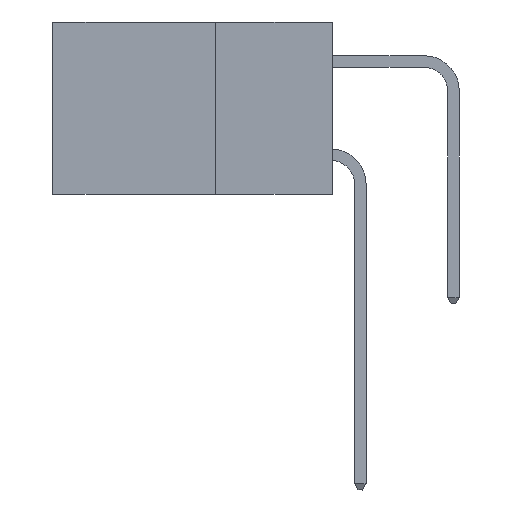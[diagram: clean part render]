
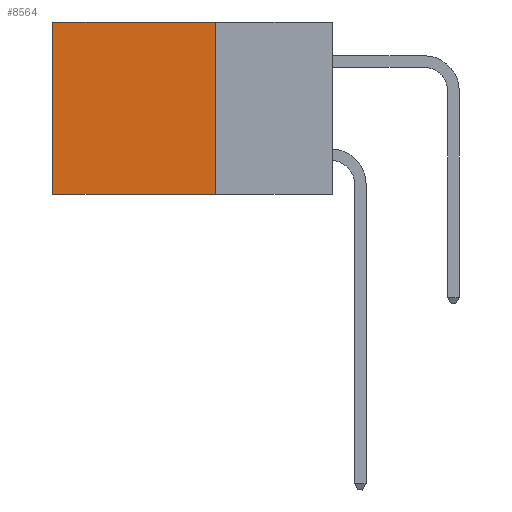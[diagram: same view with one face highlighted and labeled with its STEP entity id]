
A CAD part, left-side view. The second image highlights one B-rep face of the part: STEP entity #8564.
In plain terms, the highlighted planar face has unit normal (-1, 0, 0).
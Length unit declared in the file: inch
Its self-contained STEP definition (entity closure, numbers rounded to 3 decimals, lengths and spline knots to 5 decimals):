
#1669 = EDGE_CURVE ( 'NONE', #14055, #18018, #20801, .T. ) ;
#3012 = VERTEX_POINT ( 'NONE', #21772 ) ;
#3444 = AXIS2_PLACEMENT_3D ( 'NONE', #14337, #22350, #10398 ) ;
#4291 = PLANE ( 'NONE',  #3444 ) ;
#4457 = FACE_OUTER_BOUND ( 'NONE', #13215, .T. ) ;
#4543 = CARTESIAN_POINT ( 'NONE',  ( 0.298, 0.6, 0. ) ) ;
#6058 = CARTESIAN_POINT ( 'NONE',  ( 0.298, 0.6, -0.37 ) ) ;
#6430 = DIRECTION ( 'NONE',  ( 0., 1., 0. ) ) ;
#6864 = CARTESIAN_POINT ( 'NONE',  ( 0.298, 0.25, -0.37 ) ) ;
#7006 = LINE ( 'NONE', #14476, #21734 ) ;
#8564 = ADVANCED_FACE ( 'NONE', ( #4457 ), #4291, .F. ) ;
#8604 = EDGE_CURVE ( 'NONE', #14055, #3012, #18590, .T. ) ;
#9523 = CARTESIAN_POINT ( 'NONE',  ( 0.298, 0.25, 0. ) ) ;
#10398 = DIRECTION ( 'NONE',  ( 0., 0., -1. ) ) ;
#10543 = DIRECTION ( 'NONE',  ( 0., 1., 0. ) ) ;
#10995 = ORIENTED_EDGE ( 'NONE', *, *, #11214, .F. ) ;
#11064 = VERTEX_POINT ( 'NONE', #6058 ) ;
#11214 = EDGE_CURVE ( 'NONE', #18018, #11064, #7006, .T. ) ;
#11528 = DIRECTION ( 'NONE',  ( 0., 0., -1. ) ) ;
#11927 = ORIENTED_EDGE ( 'NONE', *, *, #1669, .F. ) ;
#12645 = VECTOR ( 'NONE', #6430, 39.37008 ) ;
#13215 = EDGE_LOOP ( 'NONE', ( #22531, #10995, #11927, #20189 ) ) ;
#14055 = VERTEX_POINT ( 'NONE', #23748 ) ;
#14337 = CARTESIAN_POINT ( 'NONE',  ( 0.298, 0.25, 0. ) ) ;
#14476 = CARTESIAN_POINT ( 'NONE',  ( 0.298, 0.25, -0.37 ) ) ;
#15146 = EDGE_CURVE ( 'NONE', #3012, #11064, #21012, .T. ) ;
#16939 = VECTOR ( 'NONE', #24494, 39.37008 ) ;
#18018 = VERTEX_POINT ( 'NONE', #6864 ) ;
#18590 = LINE ( 'NONE', #20449, #12645 ) ;
#20189 = ORIENTED_EDGE ( 'NONE', *, *, #8604, .T. ) ;
#20449 = CARTESIAN_POINT ( 'NONE',  ( 0.298, 0.25, 0. ) ) ;
#20801 = LINE ( 'NONE', #9523, #25444 ) ;
#21012 = LINE ( 'NONE', #4543, #16939 ) ;
#21734 = VECTOR ( 'NONE', #10543, 39.37008 ) ;
#21772 = CARTESIAN_POINT ( 'NONE',  ( 0.298, 0.6, 0. ) ) ;
#22350 = DIRECTION ( 'NONE',  ( 1., 0., 0. ) ) ;
#22531 = ORIENTED_EDGE ( 'NONE', *, *, #15146, .T. ) ;
#23748 = CARTESIAN_POINT ( 'NONE',  ( 0.298, 0.25, 0. ) ) ;
#24494 = DIRECTION ( 'NONE',  ( 0., 0., -1. ) ) ;
#25444 = VECTOR ( 'NONE', #11528, 39.37008 ) ;
